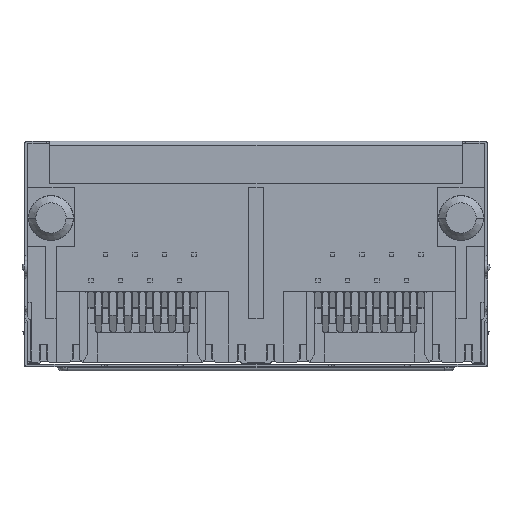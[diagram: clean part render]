
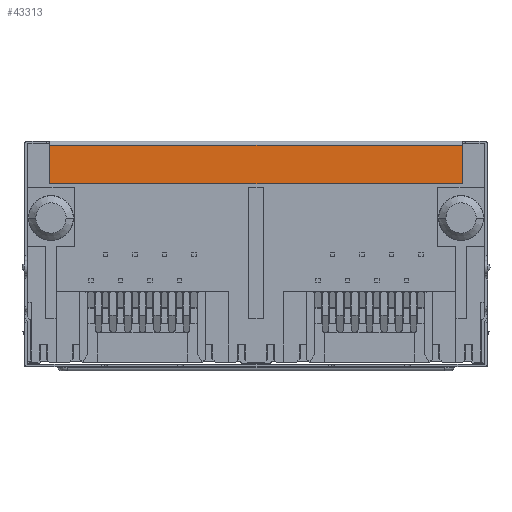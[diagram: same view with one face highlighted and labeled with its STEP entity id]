
A CAD part, front view. The second image highlights one B-rep face of the part: STEP entity #43313.
In plain terms, the highlighted planar face has unit normal (0, -1, 0).
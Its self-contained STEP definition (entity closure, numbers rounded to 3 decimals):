
#1399 = LINE ( 'NONE', #47637, #23694 ) ;
#4560 = VERTEX_POINT ( 'NONE', #44899 ) ;
#7096 = DIRECTION ( 'NONE',  ( 1., 0., 0. ) ) ;
#8722 = DIRECTION ( 'NONE',  ( 0., 0., -1. ) ) ;
#11307 = DIRECTION ( 'NONE',  ( 1., 0., 0. ) ) ;
#12104 = EDGE_LOOP ( 'NONE', ( #39343, #17601, #26454, #14564 ) ) ;
#12794 = CARTESIAN_POINT ( 'NONE',  ( 1.56, 3.84, 15.04 ) ) ;
#14564 = ORIENTED_EDGE ( 'NONE', *, *, #52484, .T. ) ;
#15419 = DIRECTION ( 'NONE',  ( 0., 0., 1. ) ) ;
#16018 = VECTOR ( 'NONE', #7096, 1000. ) ;
#17601 = ORIENTED_EDGE ( 'NONE', *, *, #50030, .F. ) ;
#19354 = CARTESIAN_POINT ( 'NONE',  ( 89.301, 3.84, 15.04 ) ) ;
#19599 = LINE ( 'NONE', #52169, #51439 ) ;
#21668 = EDGE_CURVE ( 'NONE', #37681, #40659, #46237, .T. ) ;
#21969 = CARTESIAN_POINT ( 'NONE',  ( 1.56, 3.84, 12.38 ) ) ;
#23694 = VECTOR ( 'NONE', #15419, 1000. ) ;
#26454 = ORIENTED_EDGE ( 'NONE', *, *, #21668, .T. ) ;
#28246 = AXIS2_PLACEMENT_3D ( 'NONE', #47787, #47971, #11307 ) ;
#31582 = PLANE ( 'NONE',  #28246 ) ;
#35506 = VERTEX_POINT ( 'NONE', #35938 ) ;
#35938 = CARTESIAN_POINT ( 'NONE',  ( 30.21, 3.84, 15.04 ) ) ;
#36107 = VECTOR ( 'NONE', #8722, 1000. ) ;
#37681 = VERTEX_POINT ( 'NONE', #12794 ) ;
#39343 = ORIENTED_EDGE ( 'NONE', *, *, #50072, .T. ) ;
#40659 = VERTEX_POINT ( 'NONE', #21969 ) ;
#43313 = ADVANCED_FACE ( 'NONE', ( #44954 ), #31582, .T. ) ;
#43442 = DIRECTION ( 'NONE',  ( 1., 0., 0. ) ) ;
#44899 = CARTESIAN_POINT ( 'NONE',  ( 30.21, 3.84, 12.38 ) ) ;
#44954 = FACE_OUTER_BOUND ( 'NONE', #12104, .T. ) ;
#45154 = CARTESIAN_POINT ( 'NONE',  ( 1.56, 3.84, 15.039 ) ) ;
#45941 = LINE ( 'NONE', #19354, #16018 ) ;
#46237 = LINE ( 'NONE', #45154, #36107 ) ;
#47637 = CARTESIAN_POINT ( 'NONE',  ( 30.21, 3.84, 15.039 ) ) ;
#47787 = CARTESIAN_POINT ( 'NONE',  ( 1.56, 3.84, 15.039 ) ) ;
#47971 = DIRECTION ( 'NONE',  ( 0., -1., 0. ) ) ;
#50030 = EDGE_CURVE ( 'NONE', #37681, #35506, #45941, .T. ) ;
#50072 = EDGE_CURVE ( 'NONE', #4560, #35506, #1399, .T. ) ;
#51439 = VECTOR ( 'NONE', #43442, 1000. ) ;
#52169 = CARTESIAN_POINT ( 'NONE',  ( 1.56, 3.84, 12.38 ) ) ;
#52484 = EDGE_CURVE ( 'NONE', #40659, #4560, #19599, .T. ) ;
